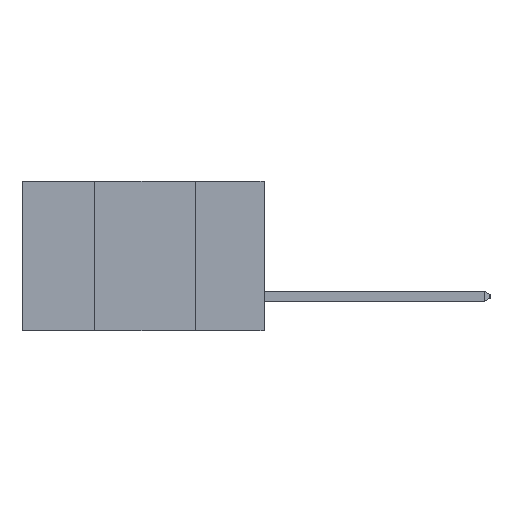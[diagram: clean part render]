
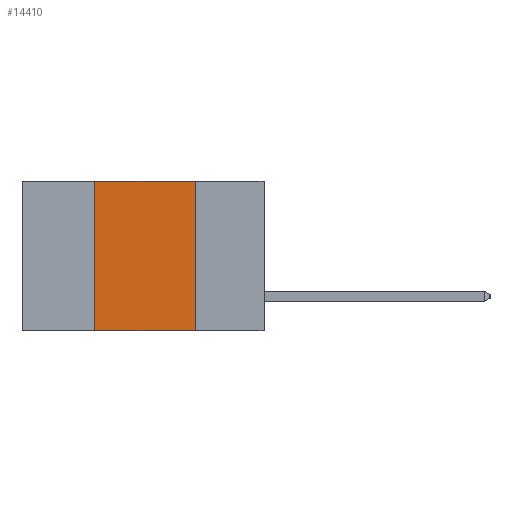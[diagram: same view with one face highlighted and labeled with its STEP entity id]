
A CAD part, left-side view. The second image highlights one B-rep face of the part: STEP entity #14410.
In plain terms, the highlighted planar face has unit normal (-1, 0, 0).
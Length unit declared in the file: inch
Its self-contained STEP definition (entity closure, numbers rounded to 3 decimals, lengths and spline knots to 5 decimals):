
#1384 = DIRECTION ( 'NONE',  ( 0., 0., -1. ) ) ;
#1770 = VERTEX_POINT ( 'NONE', #4687 ) ;
#2777 = CARTESIAN_POINT ( 'NONE',  ( 0., 0.42, -0.37 ) ) ;
#2844 = VECTOR ( 'NONE', #21322, 39.37008 ) ;
#3416 = CARTESIAN_POINT ( 'NONE',  ( 0., 0.6, 0. ) ) ;
#4628 = DIRECTION ( 'NONE',  ( 0., -1., 0. ) ) ;
#4687 = CARTESIAN_POINT ( 'NONE',  ( 0., 0.17, 0. ) ) ;
#5218 = CARTESIAN_POINT ( 'NONE',  ( 0., 0.42, 0. ) ) ;
#5255 = DIRECTION ( 'NONE',  ( 0., 0., -1. ) ) ;
#5783 = CARTESIAN_POINT ( 'NONE',  ( 0., 0.17, -0.37 ) ) ;
#6075 = AXIS2_PLACEMENT_3D ( 'NONE', #3416, #16322, #5255 ) ;
#6274 = EDGE_CURVE ( 'NONE', #1770, #20562, #20035, .T. ) ;
#7052 = VERTEX_POINT ( 'NONE', #5218 ) ;
#8403 = CARTESIAN_POINT ( 'NONE',  ( 0., 0.42, -0.37 ) ) ;
#9244 = ORIENTED_EDGE ( 'NONE', *, *, #13564, .F. ) ;
#9401 = EDGE_CURVE ( 'NONE', #11368, #7052, #22469, .T. ) ;
#10638 = PLANE ( 'NONE',  #6075 ) ;
#11357 = VECTOR ( 'NONE', #1384, 39.37008 ) ;
#11368 = VERTEX_POINT ( 'NONE', #2777 ) ;
#12653 = VECTOR ( 'NONE', #4628, 39.37008 ) ;
#13564 = EDGE_CURVE ( 'NONE', #7052, #1770, #18126, .T. ) ;
#13830 = CARTESIAN_POINT ( 'NONE',  ( 0., 0.6, 0. ) ) ;
#14410 = ADVANCED_FACE ( 'NONE', ( #22988 ), #10638, .F. ) ;
#15579 = ORIENTED_EDGE ( 'NONE', *, *, #9401, .F. ) ;
#16322 = DIRECTION ( 'NONE',  ( 1., 0., 0. ) ) ;
#16405 = VECTOR ( 'NONE', #17575, 39.37008 ) ;
#16962 = LINE ( 'NONE', #23064, #16405 ) ;
#17575 = DIRECTION ( 'NONE',  ( 0., -1., 0. ) ) ;
#17767 = ORIENTED_EDGE ( 'NONE', *, *, #20194, .T. ) ;
#18126 = LINE ( 'NONE', #13830, #12653 ) ;
#19503 = EDGE_LOOP ( 'NONE', ( #22530, #9244, #15579, #17767 ) ) ;
#19854 = CARTESIAN_POINT ( 'NONE',  ( 0., 0.17, -0.37 ) ) ;
#20035 = LINE ( 'NONE', #19854, #11357 ) ;
#20194 = EDGE_CURVE ( 'NONE', #11368, #20562, #16962, .T. ) ;
#20562 = VERTEX_POINT ( 'NONE', #5783 ) ;
#21322 = DIRECTION ( 'NONE',  ( 0., 0., 1. ) ) ;
#22469 = LINE ( 'NONE', #8403, #2844 ) ;
#22530 = ORIENTED_EDGE ( 'NONE', *, *, #6274, .F. ) ;
#22988 = FACE_OUTER_BOUND ( 'NONE', #19503, .T. ) ;
#23064 = CARTESIAN_POINT ( 'NONE',  ( 0., 0.6, -0.37 ) ) ;
